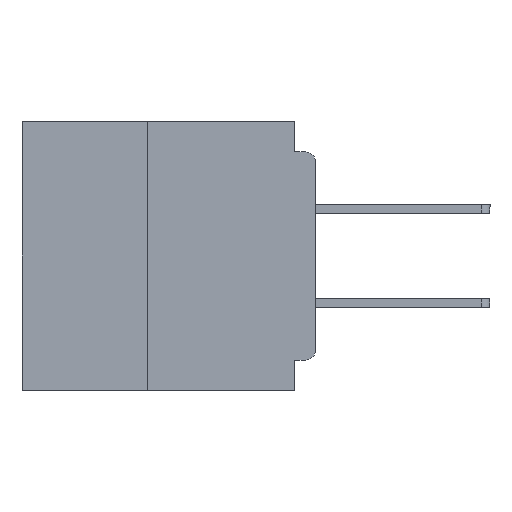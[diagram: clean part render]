
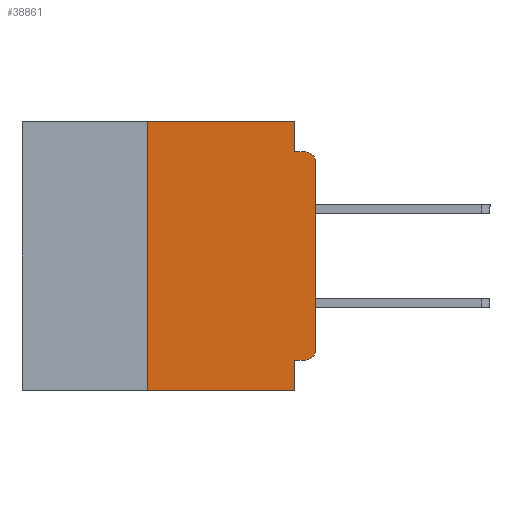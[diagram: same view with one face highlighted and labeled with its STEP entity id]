
A CAD part, left-side view. The second image highlights one B-rep face of the part: STEP entity #38861.
In plain terms, the highlighted planar face has unit normal (-1, 0, 0).
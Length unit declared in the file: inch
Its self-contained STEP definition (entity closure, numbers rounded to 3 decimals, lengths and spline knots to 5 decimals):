
#101 = ORIENTED_EDGE ( 'NONE', *, *, #21433, .T. ) ;
#262 = ORIENTED_EDGE ( 'NONE', *, *, #33537, .T. ) ;
#1331 = AXIS2_PLACEMENT_3D ( 'NONE', #14999, #42050, #18909 ) ;
#1645 = CARTESIAN_POINT ( 'NONE',  ( 0., 0., -0.06 ) ) ;
#2184 = ORIENTED_EDGE ( 'NONE', *, *, #37988, .F. ) ;
#2813 = VECTOR ( 'NONE', #39198, 39.37008 ) ;
#3262 = VERTEX_POINT ( 'NONE', #1645 ) ;
#4014 = LINE ( 'NONE', #19933, #2813 ) ;
#4475 = FACE_OUTER_BOUND ( 'NONE', #24386, .T. ) ;
#4610 = ORIENTED_EDGE ( 'NONE', *, *, #44262, .F. ) ;
#4649 = VECTOR ( 'NONE', #37123, 39.37008 ) ;
#4836 = DIRECTION ( 'NONE',  ( 0., -1., 0. ) ) ;
#7155 = CARTESIAN_POINT ( 'NONE',  ( 0., 0.031, 0. ) ) ;
#7984 = CARTESIAN_POINT ( 'NONE',  ( 0., 0.031, 0. ) ) ;
#8780 = CARTESIAN_POINT ( 'NONE',  ( 0., 0.437, -0.4 ) ) ;
#10576 = LINE ( 'NONE', #21976, #27615 ) ;
#11073 = ORIENTED_EDGE ( 'NONE', *, *, #28934, .F. ) ;
#11571 = CARTESIAN_POINT ( 'NONE',  ( 0., 0.25, 0. ) ) ;
#12877 = CARTESIAN_POINT ( 'NONE',  ( 0., 0., -0.045 ) ) ;
#13625 = EDGE_CURVE ( 'NONE', #37139, #29911, #42151, .T. ) ;
#14999 = CARTESIAN_POINT ( 'NONE',  ( 0., 0.437, 0. ) ) ;
#15060 = VERTEX_POINT ( 'NONE', #27087 ) ;
#15911 = CIRCLE ( 'NONE', #18330, 0.015 ) ;
#17596 = LINE ( 'NONE', #8780, #26734 ) ;
#18330 = AXIS2_PLACEMENT_3D ( 'NONE', #19825, #46801, #23736 ) ;
#18909 = DIRECTION ( 'NONE',  ( 0., 0., -1. ) ) ;
#19411 = LINE ( 'NONE', #40069, #49001 ) ;
#19825 = CARTESIAN_POINT ( 'NONE',  ( 0., 0.015, -0.06 ) ) ;
#19933 = CARTESIAN_POINT ( 'NONE',  ( 0., 0., 0. ) ) ;
#21109 = DIRECTION ( 'NONE',  ( -1., 0., 0. ) ) ;
#21433 = EDGE_CURVE ( 'NONE', #47340, #41502, #17596, .T. ) ;
#21976 = CARTESIAN_POINT ( 'NONE',  ( 0., 0.437, 0. ) ) ;
#22830 = EDGE_CURVE ( 'NONE', #15060, #41502, #24144, .T. ) ;
#22937 = VERTEX_POINT ( 'NONE', #37610 ) ;
#23736 = DIRECTION ( 'NONE',  ( 0., 0., -1. ) ) ;
#24071 = VECTOR ( 'NONE', #39576, 39.37008 ) ;
#24105 = CIRCLE ( 'NONE', #43014, 0.015 ) ;
#24144 = LINE ( 'NONE', #48547, #4649 ) ;
#24386 = EDGE_LOOP ( 'NONE', ( #44962, #37482, #11073, #44735, #31233, #4610, #101, #31416, #2184, #262 ) ) ;
#26734 = VECTOR ( 'NONE', #4836, 39.37008 ) ;
#27087 = CARTESIAN_POINT ( 'NONE',  ( 0., 0.031, -0.355 ) ) ;
#27572 = VECTOR ( 'NONE', #36291, 39.37008 ) ;
#27615 = VECTOR ( 'NONE', #37487, 39.37008 ) ;
#28468 = DIRECTION ( 'NONE',  ( 0., 1., 0. ) ) ;
#28496 = EDGE_CURVE ( 'NONE', #38934, #37139, #10576, .T. ) ;
#28774 = LINE ( 'NONE', #12877, #27572 ) ;
#28934 = EDGE_CURVE ( 'NONE', #29911, #22937, #28774, .T. ) ;
#29911 = VERTEX_POINT ( 'NONE', #37180 ) ;
#30698 = VECTOR ( 'NONE', #34271, 39.37008 ) ;
#31233 = ORIENTED_EDGE ( 'NONE', *, *, #28496, .F. ) ;
#31416 = ORIENTED_EDGE ( 'NONE', *, *, #22830, .F. ) ;
#33331 = EDGE_CURVE ( 'NONE', #43847, #3262, #4014, .T. ) ;
#33537 = EDGE_CURVE ( 'NONE', #44994, #43847, #24105, .T. ) ;
#34271 = DIRECTION ( 'NONE',  ( 0., 0., -1. ) ) ;
#36291 = DIRECTION ( 'NONE',  ( 0., -1., 0. ) ) ;
#37123 = DIRECTION ( 'NONE',  ( 0., 0., -1. ) ) ;
#37139 = VERTEX_POINT ( 'NONE', #7984 ) ;
#37180 = CARTESIAN_POINT ( 'NONE',  ( 0., 0.031, -0.045 ) ) ;
#37482 = ORIENTED_EDGE ( 'NONE', *, *, #40113, .T. ) ;
#37487 = DIRECTION ( 'NONE',  ( 0., -1., 0. ) ) ;
#37610 = CARTESIAN_POINT ( 'NONE',  ( 0., 0.015, -0.045 ) ) ;
#37988 = EDGE_CURVE ( 'NONE', #44994, #15060, #19411, .T. ) ;
#38861 = ADVANCED_FACE ( 'NONE', ( #4475 ), #49613, .F. ) ;
#38934 = VERTEX_POINT ( 'NONE', #11571 ) ;
#39198 = DIRECTION ( 'NONE',  ( 0., 0., 1. ) ) ;
#39576 = DIRECTION ( 'NONE',  ( 0., 0., 1. ) ) ;
#40069 = CARTESIAN_POINT ( 'NONE',  ( 0., 0., -0.355 ) ) ;
#40113 = EDGE_CURVE ( 'NONE', #3262, #22937, #15911, .T. ) ;
#40935 = CARTESIAN_POINT ( 'NONE',  ( 0., 0., -0.34 ) ) ;
#41502 = VERTEX_POINT ( 'NONE', #45530 ) ;
#42050 = DIRECTION ( 'NONE',  ( 1., 0., 0. ) ) ;
#42151 = LINE ( 'NONE', #7155, #30698 ) ;
#43014 = AXIS2_PLACEMENT_3D ( 'NONE', #44219, #21109, #48082 ) ;
#43417 = CARTESIAN_POINT ( 'NONE',  ( 0., 0.25, -0.4 ) ) ;
#43847 = VERTEX_POINT ( 'NONE', #40935 ) ;
#44219 = CARTESIAN_POINT ( 'NONE',  ( 0., 0.015, -0.34 ) ) ;
#44262 = EDGE_CURVE ( 'NONE', #47340, #38934, #44567, .T. ) ;
#44395 = CARTESIAN_POINT ( 'NONE',  ( 0., 0.25, -0.4 ) ) ;
#44567 = LINE ( 'NONE', #43417, #24071 ) ;
#44735 = ORIENTED_EDGE ( 'NONE', *, *, #13625, .F. ) ;
#44962 = ORIENTED_EDGE ( 'NONE', *, *, #33331, .T. ) ;
#44994 = VERTEX_POINT ( 'NONE', #49483 ) ;
#45530 = CARTESIAN_POINT ( 'NONE',  ( 0., 0.031, -0.4 ) ) ;
#46801 = DIRECTION ( 'NONE',  ( -1., 0., 0. ) ) ;
#47340 = VERTEX_POINT ( 'NONE', #44395 ) ;
#48082 = DIRECTION ( 'NONE',  ( 0., 0., -1. ) ) ;
#48547 = CARTESIAN_POINT ( 'NONE',  ( 0., 0.031, -0.4 ) ) ;
#49001 = VECTOR ( 'NONE', #28468, 39.37008 ) ;
#49483 = CARTESIAN_POINT ( 'NONE',  ( 0., 0.015, -0.355 ) ) ;
#49613 = PLANE ( 'NONE',  #1331 ) ;
